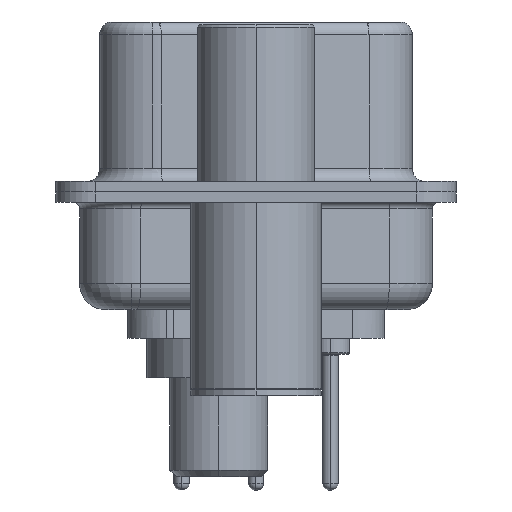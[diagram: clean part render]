
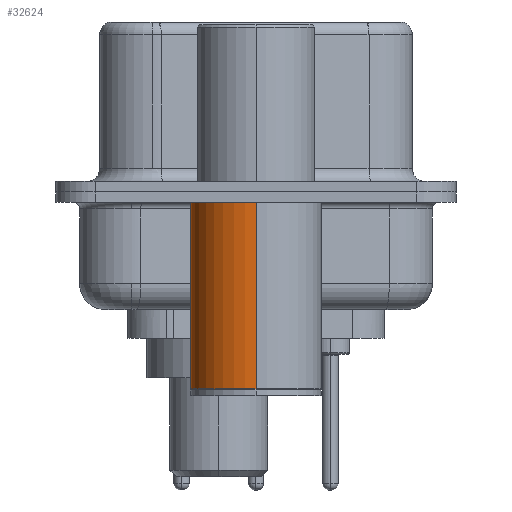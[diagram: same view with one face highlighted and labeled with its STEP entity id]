
A CAD part, left-side view. The second image highlights one B-rep face of the part: STEP entity #32624.
In plain terms, the highlighted cylindrical face has radius 2.5 mm (diameter 5 mm), a partial arc.
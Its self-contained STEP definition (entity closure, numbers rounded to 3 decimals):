
#1765 = VERTEX_POINT ( 'NONE', #14943 ) ;
#1960 = LINE ( 'NONE', #25741, #15716 ) ;
#3385 = AXIS2_PLACEMENT_3D ( 'NONE', #22966, #7590, #25538 ) ;
#3538 = CARTESIAN_POINT ( 'NONE',  ( 2.5, 0., -0.4 ) ) ;
#4460 = DIRECTION ( 'NONE',  ( 1., 0., 0. ) ) ;
#5626 = LINE ( 'NONE', #10719, #18505 ) ;
#5952 = CARTESIAN_POINT ( 'NONE',  ( 0., 0., -0.4 ) ) ;
#6678 = ORIENTED_EDGE ( 'NONE', *, *, #18250, .T. ) ;
#7590 = DIRECTION ( 'NONE',  ( 0., 0., 1. ) ) ;
#7797 = DIRECTION ( 'NONE',  ( 0., 0., 1. ) ) ;
#8596 = DIRECTION ( 'NONE',  ( 1., 0., 0. ) ) ;
#8681 = CARTESIAN_POINT ( 'NONE',  ( 2.5, 0., -7.525 ) ) ;
#8991 = ORIENTED_EDGE ( 'NONE', *, *, #25135, .T. ) ;
#9393 = AXIS2_PLACEMENT_3D ( 'NONE', #5952, #23928, #8596 ) ;
#9738 = EDGE_LOOP ( 'NONE', ( #8991, #6678, #11926, #30802 ) ) ;
#10489 = VERTEX_POINT ( 'NONE', #8681 ) ;
#10719 = CARTESIAN_POINT ( 'NONE',  ( -2.5, 0., 0.581 ) ) ;
#11926 = ORIENTED_EDGE ( 'NONE', *, *, #29242, .F. ) ;
#13472 = CIRCLE ( 'NONE', #3385, 2.5 ) ;
#13573 = CARTESIAN_POINT ( 'NONE',  ( -2.5, 0., -0.4 ) ) ;
#14233 = VERTEX_POINT ( 'NONE', #13573 ) ;
#14673 = DIRECTION ( 'NONE',  ( 0., 0., 1. ) ) ;
#14943 = CARTESIAN_POINT ( 'NONE',  ( -2.5, 0., -7.525 ) ) ;
#15716 = VECTOR ( 'NONE', #7797, 1000. ) ;
#17129 = CYLINDRICAL_SURFACE ( 'NONE', #21649, 2.5 ) ;
#17188 = EDGE_CURVE ( 'NONE', #10489, #19248, #1960, .T. ) ;
#18250 = EDGE_CURVE ( 'NONE', #1765, #14233, #5626, .T. ) ;
#18505 = VECTOR ( 'NONE', #31224, 1000. ) ;
#19248 = VERTEX_POINT ( 'NONE', #3538 ) ;
#19838 = CARTESIAN_POINT ( 'NONE',  ( 0., 0., 0.581 ) ) ;
#21649 = AXIS2_PLACEMENT_3D ( 'NONE', #19838, #14673, #4460 ) ;
#22966 = CARTESIAN_POINT ( 'NONE',  ( 0., 0., -7.525 ) ) ;
#23928 = DIRECTION ( 'NONE',  ( 0., 0., 1. ) ) ;
#25135 = EDGE_CURVE ( 'NONE', #10489, #1765, #13472, .T. ) ;
#25246 = CIRCLE ( 'NONE', #9393, 2.5 ) ;
#25538 = DIRECTION ( 'NONE',  ( 1., 0., 0. ) ) ;
#25741 = CARTESIAN_POINT ( 'NONE',  ( 2.5, 0., 0.581 ) ) ;
#29242 = EDGE_CURVE ( 'NONE', #19248, #14233, #25246, .T. ) ;
#30801 = FACE_OUTER_BOUND ( 'NONE', #9738, .T. ) ;
#30802 = ORIENTED_EDGE ( 'NONE', *, *, #17188, .F. ) ;
#31224 = DIRECTION ( 'NONE',  ( 0., 0., 1. ) ) ;
#32624 = ADVANCED_FACE ( 'NONE', ( #30801 ), #17129, .T. ) ;
